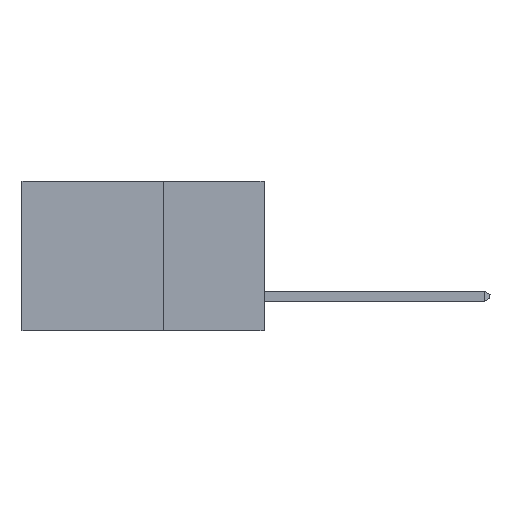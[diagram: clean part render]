
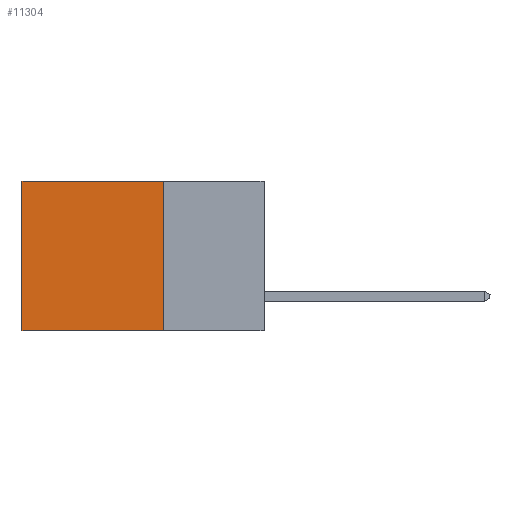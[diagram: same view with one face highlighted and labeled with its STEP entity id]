
A CAD part, left-side view. The second image highlights one B-rep face of the part: STEP entity #11304.
In plain terms, the highlighted planar face has unit normal (-1, 0, 0).
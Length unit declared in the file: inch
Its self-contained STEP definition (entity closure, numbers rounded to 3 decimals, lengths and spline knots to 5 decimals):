
#686 = DIRECTION ( 'NONE',  ( 0., 0., -1. ) ) ;
#693 = CARTESIAN_POINT ( 'NONE',  ( 0.298, 0.25, -0.37 ) ) ;
#1102 = EDGE_CURVE ( 'NONE', #11188, #9995, #5080, .T. ) ;
#2267 = LINE ( 'NONE', #7127, #5963 ) ;
#2348 = VECTOR ( 'NONE', #9044, 39.37008 ) ;
#3474 = VECTOR ( 'NONE', #7439, 39.37008 ) ;
#3703 = EDGE_CURVE ( 'NONE', #11188, #9282, #4473, .T. ) ;
#4377 = VECTOR ( 'NONE', #11499, 39.37008 ) ;
#4473 = LINE ( 'NONE', #13987, #3474 ) ;
#5080 = LINE ( 'NONE', #10093, #2348 ) ;
#5152 = EDGE_CURVE ( 'NONE', #9995, #12668, #9777, .T. ) ;
#5628 = EDGE_LOOP ( 'NONE', ( #7275, #10309, #9601, #9784 ) ) ;
#5963 = VECTOR ( 'NONE', #8222, 39.37008 ) ;
#7127 = CARTESIAN_POINT ( 'NONE',  ( 0.298, 0.6, 0. ) ) ;
#7177 = EDGE_CURVE ( 'NONE', #9282, #12668, #2267, .T. ) ;
#7185 = CARTESIAN_POINT ( 'NONE',  ( 0.298, 0.25, 0. ) ) ;
#7275 = ORIENTED_EDGE ( 'NONE', *, *, #7177, .T. ) ;
#7439 = DIRECTION ( 'NONE',  ( 0., 1., 0. ) ) ;
#7530 = FACE_OUTER_BOUND ( 'NONE', #5628, .T. ) ;
#7970 = CARTESIAN_POINT ( 'NONE',  ( 0.298, 0.25, 0. ) ) ;
#8222 = DIRECTION ( 'NONE',  ( 0., 0., -1. ) ) ;
#9044 = DIRECTION ( 'NONE',  ( 0., 0., -1. ) ) ;
#9282 = VERTEX_POINT ( 'NONE', #12016 ) ;
#9601 = ORIENTED_EDGE ( 'NONE', *, *, #1102, .F. ) ;
#9777 = LINE ( 'NONE', #12512, #4377 ) ;
#9784 = ORIENTED_EDGE ( 'NONE', *, *, #3703, .T. ) ;
#9995 = VERTEX_POINT ( 'NONE', #693 ) ;
#10093 = CARTESIAN_POINT ( 'NONE',  ( 0.298, 0.25, 0. ) ) ;
#10309 = ORIENTED_EDGE ( 'NONE', *, *, #5152, .F. ) ;
#10469 = PLANE ( 'NONE',  #10703 ) ;
#10703 = AXIS2_PLACEMENT_3D ( 'NONE', #7185, #12524, #686 ) ;
#11188 = VERTEX_POINT ( 'NONE', #7970 ) ;
#11304 = ADVANCED_FACE ( 'NONE', ( #7530 ), #10469, .F. ) ;
#11499 = DIRECTION ( 'NONE',  ( 0., 1., 0. ) ) ;
#12016 = CARTESIAN_POINT ( 'NONE',  ( 0.298, 0.6, 0. ) ) ;
#12512 = CARTESIAN_POINT ( 'NONE',  ( 0.298, 0.25, -0.37 ) ) ;
#12524 = DIRECTION ( 'NONE',  ( 1., 0., 0. ) ) ;
#12668 = VERTEX_POINT ( 'NONE', #13292 ) ;
#13292 = CARTESIAN_POINT ( 'NONE',  ( 0.298, 0.6, -0.37 ) ) ;
#13987 = CARTESIAN_POINT ( 'NONE',  ( 0.298, 0.25, 0. ) ) ;
